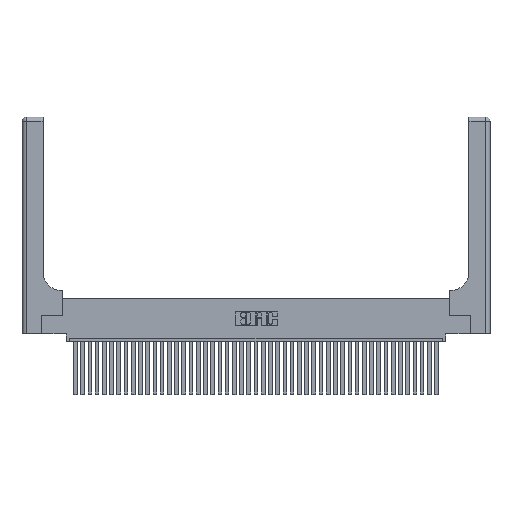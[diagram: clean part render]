
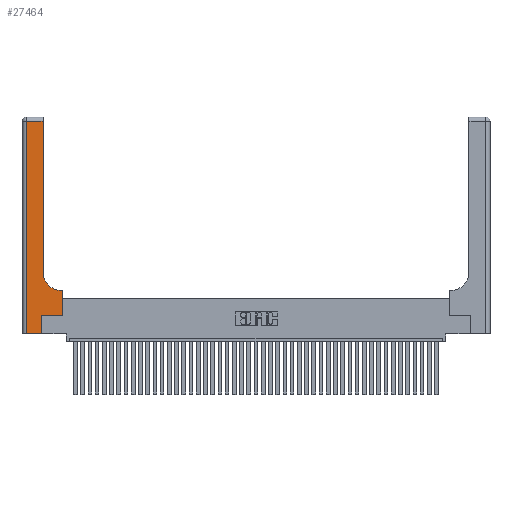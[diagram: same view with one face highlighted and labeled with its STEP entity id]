
A CAD part, top view. The second image highlights one B-rep face of the part: STEP entity #27464.
In plain terms, the highlighted planar face has unit normal (0, 0, 1).
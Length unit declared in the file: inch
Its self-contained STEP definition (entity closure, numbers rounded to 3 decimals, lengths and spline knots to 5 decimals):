
#433 = PLANE ( 'NONE',  #39806 ) ;
#967 = ORIENTED_EDGE ( 'NONE', *, *, #29691, .T. ) ;
#1264 = EDGE_CURVE ( 'NONE', #28217, #32341, #37893, .T. ) ;
#1752 = LINE ( 'NONE', #1800, #2231 ) ;
#1800 = CARTESIAN_POINT ( 'NONE',  ( 0., 0., 0.37 ) ) ;
#2231 = VECTOR ( 'NONE', #31456, 39.37008 ) ;
#3155 = VERTEX_POINT ( 'NONE', #19178 ) ;
#3323 = AXIS2_PLACEMENT_3D ( 'NONE', #30802, #8024, #14582 ) ;
#3873 = CARTESIAN_POINT ( 'NONE',  ( 0.269, 0., 0.37 ) ) ;
#4881 = FACE_OUTER_BOUND ( 'NONE', #38580, .T. ) ;
#6010 = VERTEX_POINT ( 'NONE', #24067 ) ;
#6958 = LINE ( 'NONE', #18785, #27345 ) ;
#7144 = DIRECTION ( 'NONE',  ( -1., 0., 0. ) ) ;
#7455 = ORIENTED_EDGE ( 'NONE', *, *, #33490, .T. ) ;
#8024 = DIRECTION ( 'NONE',  ( 0., 0., -1. ) ) ;
#8396 = LINE ( 'NONE', #24317, #34412 ) ;
#8733 = DIRECTION ( 'NONE',  ( 0., 1., 0. ) ) ;
#9070 = DIRECTION ( 'NONE',  ( 1., 0., 0. ) ) ;
#9307 = EDGE_CURVE ( 'NONE', #3155, #34407, #16636, .T. ) ;
#9810 = EDGE_CURVE ( 'NONE', #6010, #34180, #1752, .T. ) ;
#10691 = CARTESIAN_POINT ( 'NONE',  ( 0., 3., 0.37 ) ) ;
#11278 = VECTOR ( 'NONE', #22165, 39.37008 ) ;
#11686 = ORIENTED_EDGE ( 'NONE', *, *, #9307, .T. ) ;
#11695 = EDGE_CURVE ( 'NONE', #32341, #41779, #40857, .T. ) ;
#12519 = CARTESIAN_POINT ( 'NONE',  ( 0., 2.94, 0.37 ) ) ;
#13196 = VECTOR ( 'NONE', #8733, 39.37008 ) ;
#14513 = ORIENTED_EDGE ( 'NONE', *, *, #11695, .T. ) ;
#14582 = DIRECTION ( 'NONE',  ( 1., 0., 0. ) ) ;
#15354 = EDGE_CURVE ( 'NONE', #41779, #3155, #8396, .T. ) ;
#16636 = CIRCLE ( 'NONE', #3323, 0.25 ) ;
#18785 = CARTESIAN_POINT ( 'NONE',  ( 0.06, 3., 0.37 ) ) ;
#19113 = ORIENTED_EDGE ( 'NONE', *, *, #25480, .T. ) ;
#19163 = VECTOR ( 'NONE', #32172, 39.37008 ) ;
#19178 = CARTESIAN_POINT ( 'NONE',  ( 0.5415, 0.6, 0.37 ) ) ;
#20412 = CARTESIAN_POINT ( 'NONE',  ( 0.5585, 0.25, 0.37 ) ) ;
#20519 = CARTESIAN_POINT ( 'NONE',  ( 0.2915, 2.94, 0.37 ) ) ;
#20858 = CARTESIAN_POINT ( 'NONE',  ( 0.269, 0.25, 0.37 ) ) ;
#21539 = CARTESIAN_POINT ( 'NONE',  ( 0.2915, 3., 0.37 ) ) ;
#21651 = LINE ( 'NONE', #12519, #19163 ) ;
#21832 = LINE ( 'NONE', #21539, #13196 ) ;
#22085 = ORIENTED_EDGE ( 'NONE', *, *, #32885, .T. ) ;
#22165 = DIRECTION ( 'NONE',  ( 0., 1., 0. ) ) ;
#23490 = DIRECTION ( 'NONE',  ( -1., 0., 0. ) ) ;
#24067 = CARTESIAN_POINT ( 'NONE',  ( 0.06, 0., 0.37 ) ) ;
#24283 = CARTESIAN_POINT ( 'NONE',  ( 0.06, 2.94, 0.37 ) ) ;
#24317 = CARTESIAN_POINT ( 'NONE',  ( 0.2915, 0.6, 0.37 ) ) ;
#25057 = ORIENTED_EDGE ( 'NONE', *, *, #9810, .T. ) ;
#25480 = EDGE_CURVE ( 'NONE', #34407, #39284, #21832, .T. ) ;
#26307 = ORIENTED_EDGE ( 'NONE', *, *, #1264, .T. ) ;
#26649 = DIRECTION ( 'NONE',  ( 0., 0., -1. ) ) ;
#27345 = VECTOR ( 'NONE', #41451, 39.37008 ) ;
#27464 = ADVANCED_FACE ( 'NONE', ( #4881 ), #433, .F. ) ;
#28206 = VERTEX_POINT ( 'NONE', #24283 ) ;
#28217 = VERTEX_POINT ( 'NONE', #20858 ) ;
#28732 = CARTESIAN_POINT ( 'NONE',  ( 0.269, 0., 0.37 ) ) ;
#29182 = VECTOR ( 'NONE', #9070, 39.37008 ) ;
#29691 = EDGE_CURVE ( 'NONE', #34180, #28217, #37342, .T. ) ;
#30802 = CARTESIAN_POINT ( 'NONE',  ( 0.5415, 0.85, 0.37 ) ) ;
#31456 = DIRECTION ( 'NONE',  ( 1., 0., 0. ) ) ;
#31637 = CARTESIAN_POINT ( 'NONE',  ( 0.5585, 0.25, 0.37 ) ) ;
#32172 = DIRECTION ( 'NONE',  ( -1., 0., 0. ) ) ;
#32341 = VERTEX_POINT ( 'NONE', #31637 ) ;
#32885 = EDGE_CURVE ( 'NONE', #28206, #6010, #6958, .T. ) ;
#33490 = EDGE_CURVE ( 'NONE', #39284, #28206, #21651, .T. ) ;
#34180 = VERTEX_POINT ( 'NONE', #3873 ) ;
#34375 = CARTESIAN_POINT ( 'NONE',  ( 0.2915, 0.85, 0.37 ) ) ;
#34407 = VERTEX_POINT ( 'NONE', #34375 ) ;
#34412 = VECTOR ( 'NONE', #23490, 39.37008 ) ;
#34508 = ORIENTED_EDGE ( 'NONE', *, *, #15354, .T. ) ;
#36562 = DIRECTION ( 'NONE',  ( 0., 1., 0. ) ) ;
#36754 = VECTOR ( 'NONE', #36562, 39.37008 ) ;
#37342 = LINE ( 'NONE', #28732, #11278 ) ;
#37893 = LINE ( 'NONE', #40868, #29182 ) ;
#38580 = EDGE_LOOP ( 'NONE', ( #19113, #7455, #22085, #25057, #967, #26307, #14513, #34508, #11686 ) ) ;
#39284 = VERTEX_POINT ( 'NONE', #20519 ) ;
#39806 = AXIS2_PLACEMENT_3D ( 'NONE', #10691, #26649, #7144 ) ;
#40857 = LINE ( 'NONE', #20412, #36754 ) ;
#40868 = CARTESIAN_POINT ( 'NONE',  ( 0.269, 0.25, 0.37 ) ) ;
#41115 = CARTESIAN_POINT ( 'NONE',  ( 0.5585, 0.6, 0.37 ) ) ;
#41451 = DIRECTION ( 'NONE',  ( 0., -1., 0. ) ) ;
#41779 = VERTEX_POINT ( 'NONE', #41115 ) ;
